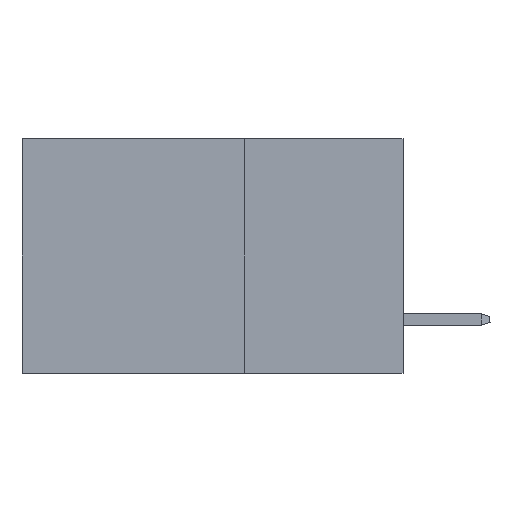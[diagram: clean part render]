
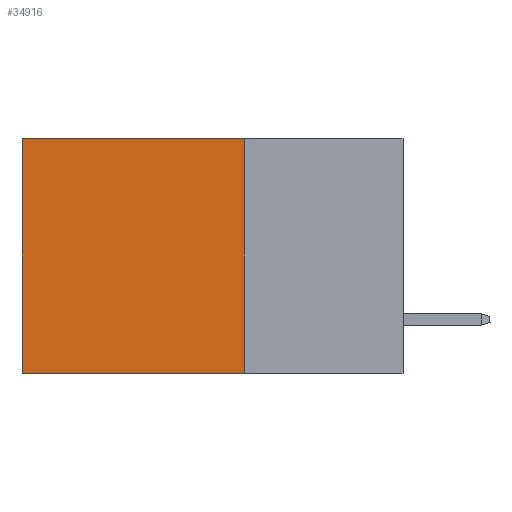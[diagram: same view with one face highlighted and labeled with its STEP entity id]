
A CAD part, left-side view. The second image highlights one B-rep face of the part: STEP entity #34916.
In plain terms, the highlighted planar face has unit normal (-1, 0, 0).
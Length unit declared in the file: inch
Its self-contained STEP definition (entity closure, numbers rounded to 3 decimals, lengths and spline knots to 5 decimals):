
#651 = VERTEX_POINT ( 'NONE', #37413 ) ;
#874 = CARTESIAN_POINT ( 'NONE',  ( 0.2875, 0.25, 0. ) ) ;
#1124 = CARTESIAN_POINT ( 'NONE',  ( 0.2875, 0.6, -0.37 ) ) ;
#1797 = CARTESIAN_POINT ( 'NONE',  ( 0.2875, 0.6, 0. ) ) ;
#2277 = ORIENTED_EDGE ( 'NONE', *, *, #12501, .F. ) ;
#2645 = VECTOR ( 'NONE', #26822, 39.37008 ) ;
#3562 = DIRECTION ( 'NONE',  ( 1., 0., 0. ) ) ;
#4005 = FACE_OUTER_BOUND ( 'NONE', #7049, .T. ) ;
#7049 = EDGE_LOOP ( 'NONE', ( #43202, #7635, #2277, #38649 ) ) ;
#7635 = ORIENTED_EDGE ( 'NONE', *, *, #27078, .F. ) ;
#8116 = VECTOR ( 'NONE', #8535, 39.37008 ) ;
#8535 = DIRECTION ( 'NONE',  ( 0., 1., 0. ) ) ;
#10595 = CARTESIAN_POINT ( 'NONE',  ( 0.2875, 0.25, 0. ) ) ;
#12501 = EDGE_CURVE ( 'NONE', #19272, #651, #13241, .T. ) ;
#13241 = LINE ( 'NONE', #37025, #29200 ) ;
#18232 = VERTEX_POINT ( 'NONE', #1124 ) ;
#18859 = EDGE_CURVE ( 'NONE', #34761, #18232, #38684, .T. ) ;
#19272 = VERTEX_POINT ( 'NONE', #41709 ) ;
#24834 = AXIS2_PLACEMENT_3D ( 'NONE', #874, #3562, #41159 ) ;
#25854 = CARTESIAN_POINT ( 'NONE',  ( 0.2875, 0.25, -0.37 ) ) ;
#26822 = DIRECTION ( 'NONE',  ( 0., 1., 0. ) ) ;
#27050 = LINE ( 'NONE', #10595, #2645 ) ;
#27078 = EDGE_CURVE ( 'NONE', #651, #18232, #28982, .T. ) ;
#27278 = VECTOR ( 'NONE', #39976, 39.37008 ) ;
#27357 = PLANE ( 'NONE',  #24834 ) ;
#28982 = LINE ( 'NONE', #25854, #8116 ) ;
#29200 = VECTOR ( 'NONE', #38302, 39.37008 ) ;
#32648 = CARTESIAN_POINT ( 'NONE',  ( 0.2875, 0.6, 0. ) ) ;
#34761 = VERTEX_POINT ( 'NONE', #1797 ) ;
#34916 = ADVANCED_FACE ( 'NONE', ( #4005 ), #27357, .F. ) ;
#37025 = CARTESIAN_POINT ( 'NONE',  ( 0.2875, 0.25, 0. ) ) ;
#37413 = CARTESIAN_POINT ( 'NONE',  ( 0.2875, 0.25, -0.37 ) ) ;
#38302 = DIRECTION ( 'NONE',  ( 0., 0., -1. ) ) ;
#38649 = ORIENTED_EDGE ( 'NONE', *, *, #43788, .T. ) ;
#38684 = LINE ( 'NONE', #32648, #27278 ) ;
#39976 = DIRECTION ( 'NONE',  ( 0., 0., -1. ) ) ;
#41159 = DIRECTION ( 'NONE',  ( 0., 0., -1. ) ) ;
#41709 = CARTESIAN_POINT ( 'NONE',  ( 0.2875, 0.25, 0. ) ) ;
#43202 = ORIENTED_EDGE ( 'NONE', *, *, #18859, .T. ) ;
#43788 = EDGE_CURVE ( 'NONE', #19272, #34761, #27050, .T. ) ;
